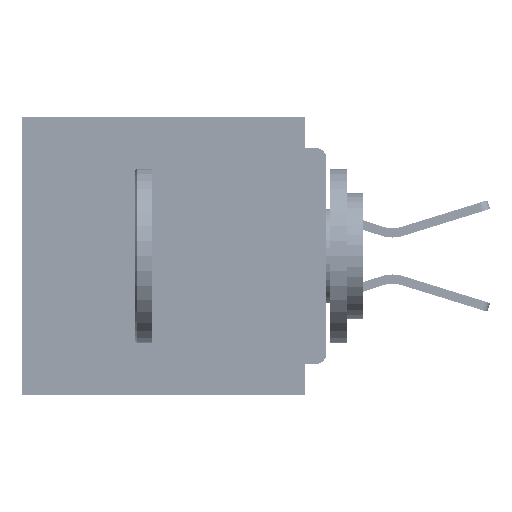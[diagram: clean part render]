
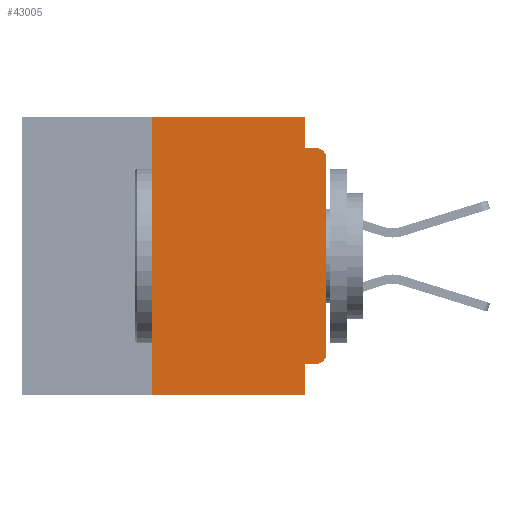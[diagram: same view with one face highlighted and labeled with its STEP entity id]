
A CAD part, left-side view. The second image highlights one B-rep face of the part: STEP entity #43005.
In plain terms, the highlighted planar face has unit normal (-1, 0, 0).
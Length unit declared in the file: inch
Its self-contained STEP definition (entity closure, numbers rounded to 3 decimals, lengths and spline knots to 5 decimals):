
#970 = DIRECTION ( 'NONE',  ( -1., 0., 0. ) ) ;
#1304 = VECTOR ( 'NONE', #36196, 39.37008 ) ;
#1588 = VERTEX_POINT ( 'NONE', #11625 ) ;
#1969 = VERTEX_POINT ( 'NONE', #54543 ) ;
#2791 = DIRECTION ( 'NONE',  ( 1., 0., 0. ) ) ;
#3142 = ORIENTED_EDGE ( 'NONE', *, *, #63010, .T. ) ;
#4351 = CARTESIAN_POINT ( 'NONE',  ( 0., 0.437, 0. ) ) ;
#4782 = CARTESIAN_POINT ( 'NONE',  ( 0., 0.25, -0.4 ) ) ;
#5822 = DIRECTION ( 'NONE',  ( 0., 0., 1. ) ) ;
#8283 = AXIS2_PLACEMENT_3D ( 'NONE', #32059, #970, #37283 ) ;
#9098 = VERTEX_POINT ( 'NONE', #25537 ) ;
#10097 = DIRECTION ( 'NONE',  ( 0., 0., 1. ) ) ;
#10904 = AXIS2_PLACEMENT_3D ( 'NONE', #23480, #2791, #39131 ) ;
#11625 = CARTESIAN_POINT ( 'NONE',  ( 0., 0., -0.34 ) ) ;
#13084 = CARTESIAN_POINT ( 'NONE',  ( 0., 0., -0.355 ) ) ;
#13541 = DIRECTION ( 'NONE',  ( 0., 0., -1. ) ) ;
#14589 = VECTOR ( 'NONE', #21346, 39.37008 ) ;
#15067 = CARTESIAN_POINT ( 'NONE',  ( 0., 0.031, -0.4 ) ) ;
#15196 = LINE ( 'NONE', #61997, #1304 ) ;
#16159 = CARTESIAN_POINT ( 'NONE',  ( 0., 0., -0.045 ) ) ;
#18271 = DIRECTION ( 'NONE',  ( 0., 1., 0. ) ) ;
#19697 = EDGE_CURVE ( 'NONE', #50723, #35546, #39901, .T. ) ;
#21346 = DIRECTION ( 'NONE',  ( 0., -1., 0. ) ) ;
#21543 = VECTOR ( 'NONE', #35416, 39.37008 ) ;
#23480 = CARTESIAN_POINT ( 'NONE',  ( 0., 0.437, 0. ) ) ;
#23897 = ORIENTED_EDGE ( 'NONE', *, *, #19697, .F. ) ;
#25520 = DIRECTION ( 'NONE',  ( -1., 0., 0. ) ) ;
#25537 = CARTESIAN_POINT ( 'NONE',  ( 0., 0.031, -0.045 ) ) ;
#26042 = ORIENTED_EDGE ( 'NONE', *, *, #45420, .F. ) ;
#26520 = ORIENTED_EDGE ( 'NONE', *, *, #29254, .T. ) ;
#27466 = CARTESIAN_POINT ( 'NONE',  ( 0., 0.015, -0.355 ) ) ;
#27696 = LINE ( 'NONE', #4782, #38229 ) ;
#27840 = EDGE_CURVE ( 'NONE', #35546, #30087, #60648, .T. ) ;
#28468 = VERTEX_POINT ( 'NONE', #44729 ) ;
#28700 = PLANE ( 'NONE',  #10904 ) ;
#29005 = LINE ( 'NONE', #32592, #41219 ) ;
#29254 = EDGE_CURVE ( 'NONE', #29666, #30087, #15196, .T. ) ;
#29666 = VERTEX_POINT ( 'NONE', #39325 ) ;
#30069 = EDGE_CURVE ( 'NONE', #1969, #28468, #45877, .T. ) ;
#30087 = VERTEX_POINT ( 'NONE', #15067 ) ;
#31869 = CARTESIAN_POINT ( 'NONE',  ( 0., 0., 0. ) ) ;
#31910 = CARTESIAN_POINT ( 'NONE',  ( 0., 0.031, -0.355 ) ) ;
#32059 = CARTESIAN_POINT ( 'NONE',  ( 0., 0.015, -0.34 ) ) ;
#32592 = CARTESIAN_POINT ( 'NONE',  ( 0., 0.031, 0. ) ) ;
#32825 = EDGE_CURVE ( 'NONE', #28468, #9098, #29005, .T. ) ;
#32952 = CIRCLE ( 'NONE', #8283, 0.015 ) ;
#35416 = DIRECTION ( 'NONE',  ( 0., -1., 0. ) ) ;
#35546 = VERTEX_POINT ( 'NONE', #31910 ) ;
#36020 = VECTOR ( 'NONE', #5822, 39.37008 ) ;
#36196 = DIRECTION ( 'NONE',  ( 0., -1., 0. ) ) ;
#37283 = DIRECTION ( 'NONE',  ( 0., 0., -1. ) ) ;
#37999 = EDGE_CURVE ( 'NONE', #29666, #1969, #27696, .T. ) ;
#38229 = VECTOR ( 'NONE', #10097, 39.37008 ) ;
#38417 = VERTEX_POINT ( 'NONE', #54641 ) ;
#38861 = LINE ( 'NONE', #16159, #14589 ) ;
#39131 = DIRECTION ( 'NONE',  ( 0., 0., -1. ) ) ;
#39325 = CARTESIAN_POINT ( 'NONE',  ( 0., 0.25, -0.4 ) ) ;
#39901 = LINE ( 'NONE', #13084, #65737 ) ;
#41219 = VECTOR ( 'NONE', #53490, 39.37008 ) ;
#43005 = ADVANCED_FACE ( 'NONE', ( #61113 ), #28700, .F. ) ;
#44128 = CIRCLE ( 'NONE', #60798, 0.015 ) ;
#44172 = CARTESIAN_POINT ( 'NONE',  ( 0., 0., -0.06 ) ) ;
#44572 = CARTESIAN_POINT ( 'NONE',  ( 0., 0.031, -0.4 ) ) ;
#44729 = CARTESIAN_POINT ( 'NONE',  ( 0., 0.031, 0. ) ) ;
#45420 = EDGE_CURVE ( 'NONE', #9098, #38417, #38861, .T. ) ;
#45877 = LINE ( 'NONE', #4351, #21543 ) ;
#45975 = EDGE_LOOP ( 'NONE', ( #61316, #47288, #26042, #54418, #55862, #50120, #26520, #55826, #23897, #3142 ) ) ;
#47288 = ORIENTED_EDGE ( 'NONE', *, *, #64553, .T. ) ;
#48997 = EDGE_CURVE ( 'NONE', #1588, #64341, #65132, .T. ) ;
#50120 = ORIENTED_EDGE ( 'NONE', *, *, #37999, .F. ) ;
#50723 = VERTEX_POINT ( 'NONE', #27466 ) ;
#53490 = DIRECTION ( 'NONE',  ( 0., 0., -1. ) ) ;
#54418 = ORIENTED_EDGE ( 'NONE', *, *, #32825, .F. ) ;
#54543 = CARTESIAN_POINT ( 'NONE',  ( 0., 0.25, 0. ) ) ;
#54641 = CARTESIAN_POINT ( 'NONE',  ( 0., 0.015, -0.045 ) ) ;
#55826 = ORIENTED_EDGE ( 'NONE', *, *, #27840, .F. ) ;
#55862 = ORIENTED_EDGE ( 'NONE', *, *, #30069, .F. ) ;
#56597 = CARTESIAN_POINT ( 'NONE',  ( 0., 0.015, -0.06 ) ) ;
#60648 = LINE ( 'NONE', #44572, #62255 ) ;
#60798 = AXIS2_PLACEMENT_3D ( 'NONE', #56597, #25520, #61758 ) ;
#61113 = FACE_OUTER_BOUND ( 'NONE', #45975, .T. ) ;
#61316 = ORIENTED_EDGE ( 'NONE', *, *, #48997, .T. ) ;
#61758 = DIRECTION ( 'NONE',  ( 0., 0., -1. ) ) ;
#61997 = CARTESIAN_POINT ( 'NONE',  ( 0., 0.437, -0.4 ) ) ;
#62255 = VECTOR ( 'NONE', #13541, 39.37008 ) ;
#63010 = EDGE_CURVE ( 'NONE', #50723, #1588, #32952, .T. ) ;
#64341 = VERTEX_POINT ( 'NONE', #44172 ) ;
#64553 = EDGE_CURVE ( 'NONE', #64341, #38417, #44128, .T. ) ;
#65132 = LINE ( 'NONE', #31869, #36020 ) ;
#65737 = VECTOR ( 'NONE', #18271, 39.37008 ) ;
